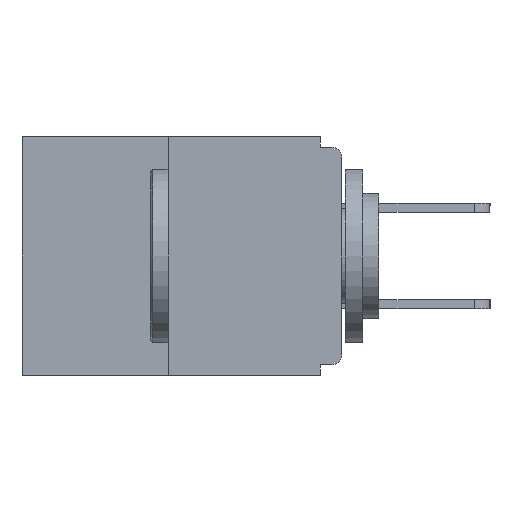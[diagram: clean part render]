
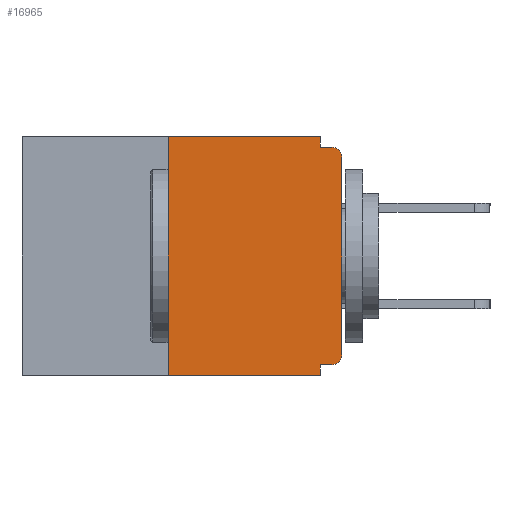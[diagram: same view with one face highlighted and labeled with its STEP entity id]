
A CAD part, left-side view. The second image highlights one B-rep face of the part: STEP entity #16965.
In plain terms, the highlighted planar face has unit normal (-1, 0, 0).
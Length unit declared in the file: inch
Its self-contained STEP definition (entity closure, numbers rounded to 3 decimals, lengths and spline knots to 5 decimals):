
#417 = CARTESIAN_POINT ( 'NONE',  ( 0., 0., 0. ) ) ;
#533 = CARTESIAN_POINT ( 'NONE',  ( 0., 0.031, -0.328 ) ) ;
#937 = CARTESIAN_POINT ( 'NONE',  ( 0., 0.031, -0.015 ) ) ;
#1005 = CARTESIAN_POINT ( 'NONE',  ( 0., 0.015, -0.015 ) ) ;
#1009 = CARTESIAN_POINT ( 'NONE',  ( 0., 0.015, -0.328 ) ) ;
#1837 = CARTESIAN_POINT ( 'NONE',  ( 0., 0.015, -0.313 ) ) ;
#2102 = LINE ( 'NONE', #7465, #20711 ) ;
#2220 = ORIENTED_EDGE ( 'NONE', *, *, #7707, .F. ) ;
#2358 = VERTEX_POINT ( 'NONE', #13622 ) ;
#2495 = VERTEX_POINT ( 'NONE', #1005 ) ;
#2549 = LINE ( 'NONE', #417, #4394 ) ;
#2667 = CARTESIAN_POINT ( 'NONE',  ( 0., 0.25, 0. ) ) ;
#3046 = VECTOR ( 'NONE', #15773, 39.37008 ) ;
#3287 = ORIENTED_EDGE ( 'NONE', *, *, #14177, .F. ) ;
#3682 = AXIS2_PLACEMENT_3D ( 'NONE', #1837, #10799, #10585 ) ;
#4004 = DIRECTION ( 'NONE',  ( 1., 0., 0. ) ) ;
#4083 = CARTESIAN_POINT ( 'NONE',  ( 0., 0., -0.03 ) ) ;
#4287 = ORIENTED_EDGE ( 'NONE', *, *, #4918, .T. ) ;
#4333 = VERTEX_POINT ( 'NONE', #9941 ) ;
#4394 = VECTOR ( 'NONE', #17105, 39.37008 ) ;
#4474 = EDGE_LOOP ( 'NONE', ( #20864, #17918, #4287, #10543, #2220, #6545, #17144, #16407, #3287, #20160 ) ) ;
#4551 = VECTOR ( 'NONE', #7594, 39.37008 ) ;
#4656 = EDGE_CURVE ( 'NONE', #8064, #11758, #5418, .T. ) ;
#4856 = DIRECTION ( 'NONE',  ( 0., -1., 0. ) ) ;
#4918 = EDGE_CURVE ( 'NONE', #8064, #4333, #2102, .T. ) ;
#4925 = VERTEX_POINT ( 'NONE', #937 ) ;
#5418 = LINE ( 'NONE', #11504, #13670 ) ;
#6511 = EDGE_CURVE ( 'NONE', #2358, #16763, #2549, .T. ) ;
#6545 = ORIENTED_EDGE ( 'NONE', *, *, #7801, .T. ) ;
#6602 = CARTESIAN_POINT ( 'NONE',  ( 0., 0., -0.015 ) ) ;
#6974 = CARTESIAN_POINT ( 'NONE',  ( 0., 0.031, 0. ) ) ;
#6996 = VERTEX_POINT ( 'NONE', #533 ) ;
#7043 = EDGE_CURVE ( 'NONE', #11758, #13534, #10371, .T. ) ;
#7380 = DIRECTION ( 'NONE',  ( 0., 0., -1. ) ) ;
#7465 = CARTESIAN_POINT ( 'NONE',  ( 0., 0.46, -0.343 ) ) ;
#7594 = DIRECTION ( 'NONE',  ( 0., 0., -1. ) ) ;
#7707 = EDGE_CURVE ( 'NONE', #13482, #6996, #19107, .T. ) ;
#7801 = EDGE_CURVE ( 'NONE', #13482, #2358, #15232, .T. ) ;
#7815 = EDGE_CURVE ( 'NONE', #13534, #4925, #19356, .T. ) ;
#8064 = VERTEX_POINT ( 'NONE', #10925 ) ;
#8270 = DIRECTION ( 'NONE',  ( 0., 0., 1. ) ) ;
#8803 = VECTOR ( 'NONE', #15448, 39.37008 ) ;
#8806 = DIRECTION ( 'NONE',  ( -1., 0., 0. ) ) ;
#9820 = EDGE_CURVE ( 'NONE', #6996, #4333, #13850, .T. ) ;
#9941 = CARTESIAN_POINT ( 'NONE',  ( 0., 0.031, -0.343 ) ) ;
#10371 = LINE ( 'NONE', #10751, #3046 ) ;
#10483 = CARTESIAN_POINT ( 'NONE',  ( 0., 0.015, -0.03 ) ) ;
#10543 = ORIENTED_EDGE ( 'NONE', *, *, #9820, .F. ) ;
#10585 = DIRECTION ( 'NONE',  ( 0., 0., -1. ) ) ;
#10751 = CARTESIAN_POINT ( 'NONE',  ( 0., 0.46, 0. ) ) ;
#10799 = DIRECTION ( 'NONE',  ( -1., 0., 0. ) ) ;
#10925 = CARTESIAN_POINT ( 'NONE',  ( 0., 0.25, -0.343 ) ) ;
#11041 = LINE ( 'NONE', #6602, #13350 ) ;
#11504 = CARTESIAN_POINT ( 'NONE',  ( 0., 0.25, 0. ) ) ;
#11592 = EDGE_CURVE ( 'NONE', #16763, #2495, #12949, .T. ) ;
#11758 = VERTEX_POINT ( 'NONE', #2667 ) ;
#11898 = AXIS2_PLACEMENT_3D ( 'NONE', #10483, #8806, #13757 ) ;
#12119 = AXIS2_PLACEMENT_3D ( 'NONE', #13914, #4004, #7380 ) ;
#12949 = CIRCLE ( 'NONE', #11898, 0.015 ) ;
#13226 = DIRECTION ( 'NONE',  ( 0., 1., 0. ) ) ;
#13350 = VECTOR ( 'NONE', #4856, 39.37008 ) ;
#13482 = VERTEX_POINT ( 'NONE', #1009 ) ;
#13534 = VERTEX_POINT ( 'NONE', #6974 ) ;
#13622 = CARTESIAN_POINT ( 'NONE',  ( 0., 0., -0.313 ) ) ;
#13627 = CARTESIAN_POINT ( 'NONE',  ( 0., 0.031, -0.343 ) ) ;
#13670 = VECTOR ( 'NONE', #8270, 39.37008 ) ;
#13757 = DIRECTION ( 'NONE',  ( 0., 0., -1. ) ) ;
#13850 = LINE ( 'NONE', #13627, #4551 ) ;
#13914 = CARTESIAN_POINT ( 'NONE',  ( 0., 0.46, 0. ) ) ;
#14177 = EDGE_CURVE ( 'NONE', #4925, #2495, #11041, .T. ) ;
#14286 = DIRECTION ( 'NONE',  ( 0., -1., 0. ) ) ;
#15232 = CIRCLE ( 'NONE', #3682, 0.015 ) ;
#15448 = DIRECTION ( 'NONE',  ( 0., 0., -1. ) ) ;
#15773 = DIRECTION ( 'NONE',  ( 0., -1., 0. ) ) ;
#16407 = ORIENTED_EDGE ( 'NONE', *, *, #11592, .T. ) ;
#16521 = VECTOR ( 'NONE', #13226, 39.37008 ) ;
#16763 = VERTEX_POINT ( 'NONE', #4083 ) ;
#16965 = ADVANCED_FACE ( 'NONE', ( #17889 ), #19039, .F. ) ;
#17105 = DIRECTION ( 'NONE',  ( 0., 0., 1. ) ) ;
#17144 = ORIENTED_EDGE ( 'NONE', *, *, #6511, .T. ) ;
#17889 = FACE_OUTER_BOUND ( 'NONE', #4474, .T. ) ;
#17918 = ORIENTED_EDGE ( 'NONE', *, *, #4656, .F. ) ;
#19039 = PLANE ( 'NONE',  #12119 ) ;
#19107 = LINE ( 'NONE', #19779, #16521 ) ;
#19356 = LINE ( 'NONE', #20265, #8803 ) ;
#19779 = CARTESIAN_POINT ( 'NONE',  ( 0., 0., -0.328 ) ) ;
#20160 = ORIENTED_EDGE ( 'NONE', *, *, #7815, .F. ) ;
#20265 = CARTESIAN_POINT ( 'NONE',  ( 0., 0.031, 0. ) ) ;
#20711 = VECTOR ( 'NONE', #14286, 39.37008 ) ;
#20864 = ORIENTED_EDGE ( 'NONE', *, *, #7043, .F. ) ;
